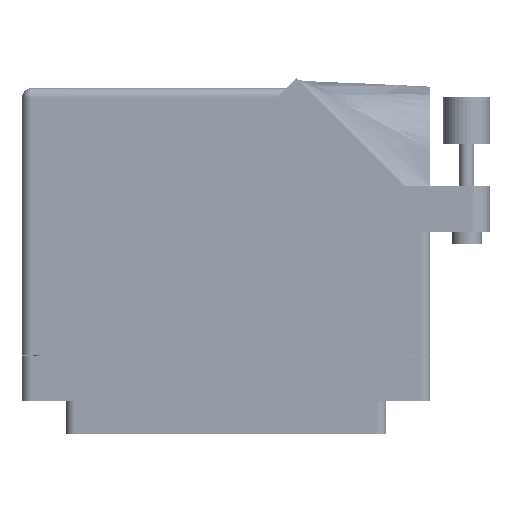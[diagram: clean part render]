
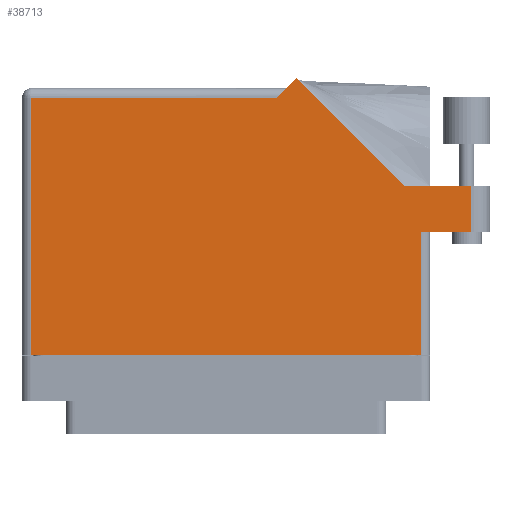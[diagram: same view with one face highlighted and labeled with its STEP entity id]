
A CAD part, front view. The second image highlights one B-rep face of the part: STEP entity #38713.
In plain terms, the highlighted face is planar.
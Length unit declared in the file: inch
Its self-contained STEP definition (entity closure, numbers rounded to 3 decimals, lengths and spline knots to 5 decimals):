
#981 = DIRECTION ( 'NONE',  ( -0.707, -0.707, 0. ) ) ;
#1479 = CARTESIAN_POINT ( 'NONE',  ( 0.399, 1.675, 0.617 ) ) ;
#2718 = CARTESIAN_POINT ( 'NONE',  ( 1.297, 0.715, 0.617 ) ) ;
#7183 = EDGE_CURVE ( 'NONE', #19140, #63134, #70778, .T. ) ;
#8543 = LINE ( 'NONE', #54706, #71868 ) ;
#8553 = LINE ( 'NONE', #32420, #12150 ) ;
#8616 = DIRECTION ( 'NONE',  ( -1., 0., 0. ) ) ;
#10440 = VECTOR ( 'NONE', #8616, 39.37008 ) ;
#12150 = VECTOR ( 'NONE', #15760, 39.37008 ) ;
#14527 = AXIS2_PLACEMENT_3D ( 'NONE', #58313, #68744, #69244 ) ;
#14589 = EDGE_CURVE ( 'NONE', #21180, #20111, #24394, .T. ) ;
#15753 = VERTEX_POINT ( 'NONE', #30633 ) ;
#15760 = DIRECTION ( 'NONE',  ( -0.707, 0.707, 0. ) ) ;
#16057 = ORIENTED_EDGE ( 'NONE', *, *, #48361, .T. ) ;
#18016 = LINE ( 'NONE', #26547, #23357 ) ;
#19140 = VERTEX_POINT ( 'NONE', #2718 ) ;
#20111 = VERTEX_POINT ( 'NONE', #43433 ) ;
#20299 = LINE ( 'NONE', #21352, #21229 ) ;
#20385 = DIRECTION ( 'NONE',  ( 0., -1., 0. ) ) ;
#21037 = LINE ( 'NONE', #1479, #49649 ) ;
#21180 = VERTEX_POINT ( 'NONE', #25154 ) ;
#21229 = VECTOR ( 'NONE', #20385, 39.37008 ) ;
#21352 = CARTESIAN_POINT ( 'NONE',  ( -1.297, -0.1, 0.617 ) ) ;
#23357 = VECTOR ( 'NONE', #72197, 39.37008 ) ;
#23801 = DIRECTION ( 'NONE',  ( 1., 0., 0. ) ) ;
#24346 = ORIENTED_EDGE ( 'NONE', *, *, #30823, .T. ) ;
#24394 = LINE ( 'NONE', #51978, #64583 ) ;
#25154 = CARTESIAN_POINT ( 'NONE',  ( -1.297, -0.1, 0.617 ) ) ;
#25185 = VECTOR ( 'NONE', #41752, 39.37008 ) ;
#26547 = CARTESIAN_POINT ( 'NONE',  ( 1.634, 1.022, 0.617 ) ) ;
#27251 = ORIENTED_EDGE ( 'NONE', *, *, #14589, .T. ) ;
#28183 = VERTEX_POINT ( 'NONE', #34104 ) ;
#30358 = ORIENTED_EDGE ( 'NONE', *, *, #67359, .T. ) ;
#30633 = CARTESIAN_POINT ( 'NONE',  ( -1.297, 1.613, 0.617 ) ) ;
#30823 = EDGE_CURVE ( 'NONE', #54831, #15753, #31443, .T. ) ;
#31443 = LINE ( 'NONE', #69455, #25185 ) ;
#32420 = CARTESIAN_POINT ( 'NONE',  ( 1.19342, 1.022, 0.617 ) ) ;
#32753 = LINE ( 'NONE', #71465, #10440 ) ;
#33307 = VECTOR ( 'NONE', #23801, 39.37008 ) ;
#33726 = EDGE_CURVE ( 'NONE', #15753, #21180, #20299, .T. ) ;
#34104 = CARTESIAN_POINT ( 'NONE',  ( 0.46971, 1.74571, 0.617 ) ) ;
#34595 = CARTESIAN_POINT ( 'NONE',  ( 1.19342, 1.022, 0.617 ) ) ;
#35174 = CARTESIAN_POINT ( 'NONE',  ( 1.634, 0.715, 0.617 ) ) ;
#35357 = PLANE ( 'NONE',  #14527 ) ;
#37921 = DIRECTION ( 'NONE',  ( 0., 1., 0. ) ) ;
#38713 = ADVANCED_FACE ( 'NONE', ( #40694 ), #35357, .F. ) ;
#38956 = EDGE_CURVE ( 'NONE', #20111, #19140, #8543, .T. ) ;
#40694 = FACE_OUTER_BOUND ( 'NONE', #51956, .T. ) ;
#40764 = CARTESIAN_POINT ( 'NONE',  ( 0.337, 1.613, 0.617 ) ) ;
#41752 = DIRECTION ( 'NONE',  ( -1., 0., 0. ) ) ;
#43433 = CARTESIAN_POINT ( 'NONE',  ( 1.297, -0.1, 0.617 ) ) ;
#48361 = EDGE_CURVE ( 'NONE', #63134, #70904, #18016, .T. ) ;
#49649 = VECTOR ( 'NONE', #981, 39.37008 ) ;
#50232 = ORIENTED_EDGE ( 'NONE', *, *, #59210, .T. ) ;
#51956 = EDGE_LOOP ( 'NONE', ( #69184, #16057, #50232, #62793, #30358, #24346, #58564, #27251, #72248 ) ) ;
#51978 = CARTESIAN_POINT ( 'NONE',  ( -1.359, -0.1, 0.617 ) ) ;
#54706 = CARTESIAN_POINT ( 'NONE',  ( 1.297, 0.715, 0.617 ) ) ;
#54831 = VERTEX_POINT ( 'NONE', #40764 ) ;
#58067 = CARTESIAN_POINT ( 'NONE',  ( 1.359, 0.715, 0.617 ) ) ;
#58313 = CARTESIAN_POINT ( 'NONE',  ( -1.359, 1.675, 0.617 ) ) ;
#58564 = ORIENTED_EDGE ( 'NONE', *, *, #33726, .T. ) ;
#59210 = EDGE_CURVE ( 'NONE', #70904, #68257, #32753, .T. ) ;
#62793 = ORIENTED_EDGE ( 'NONE', *, *, #66798, .T. ) ;
#63134 = VERTEX_POINT ( 'NONE', #35174 ) ;
#64583 = VECTOR ( 'NONE', #68106, 39.37008 ) ;
#66798 = EDGE_CURVE ( 'NONE', #68257, #28183, #8553, .T. ) ;
#67359 = EDGE_CURVE ( 'NONE', #28183, #54831, #21037, .T. ) ;
#68106 = DIRECTION ( 'NONE',  ( 1., 0., 0. ) ) ;
#68257 = VERTEX_POINT ( 'NONE', #34595 ) ;
#68744 = DIRECTION ( 'NONE',  ( 0., 0., -1. ) ) ;
#69184 = ORIENTED_EDGE ( 'NONE', *, *, #7183, .T. ) ;
#69244 = DIRECTION ( 'NONE',  ( -1., 0., 0. ) ) ;
#69259 = CARTESIAN_POINT ( 'NONE',  ( 1.634, 1.022, 0.617 ) ) ;
#69455 = CARTESIAN_POINT ( 'NONE',  ( -1.359, 1.613, 0.617 ) ) ;
#70778 = LINE ( 'NONE', #58067, #33307 ) ;
#70904 = VERTEX_POINT ( 'NONE', #69259 ) ;
#71465 = CARTESIAN_POINT ( 'NONE',  ( 1.759, 1.022, 0.617 ) ) ;
#71868 = VECTOR ( 'NONE', #37921, 39.37008 ) ;
#72197 = DIRECTION ( 'NONE',  ( 0., 1., 0. ) ) ;
#72248 = ORIENTED_EDGE ( 'NONE', *, *, #38956, .T. ) ;
